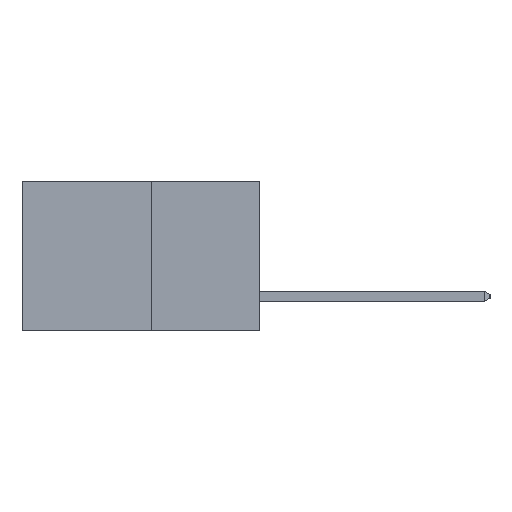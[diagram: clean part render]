
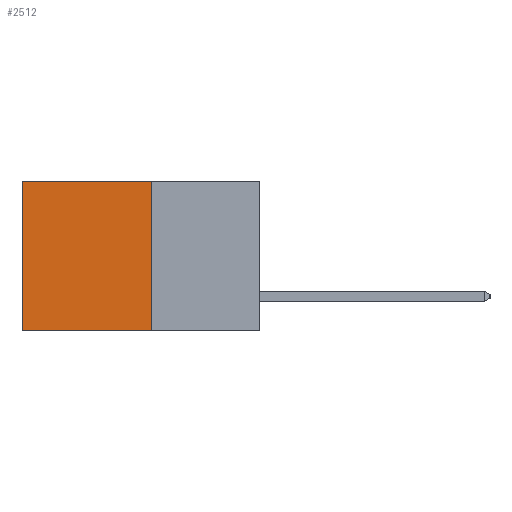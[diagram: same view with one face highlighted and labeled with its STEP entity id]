
A CAD part, left-side view. The second image highlights one B-rep face of the part: STEP entity #2512.
In plain terms, the highlighted planar face has unit normal (-1, 0, 0).
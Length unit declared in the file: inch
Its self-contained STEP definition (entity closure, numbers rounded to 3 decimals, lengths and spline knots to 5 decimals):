
#58 = VERTEX_POINT ( 'NONE', #10899 ) ;
#390 = ORIENTED_EDGE ( 'NONE', *, *, #5975, .T. ) ;
#1043 = VERTEX_POINT ( 'NONE', #5877 ) ;
#1537 = EDGE_CURVE ( 'NONE', #4087, #1043, #2656, .T. ) ;
#1836 = CARTESIAN_POINT ( 'NONE',  ( 0.277, 0.27, -0.37 ) ) ;
#1983 = FACE_OUTER_BOUND ( 'NONE', #2102, .T. ) ;
#2102 = EDGE_LOOP ( 'NONE', ( #390, #5267, #7483, #3284 ) ) ;
#2512 = ADVANCED_FACE ( 'NONE', ( #1983 ), #8039, .F. ) ;
#2656 = LINE ( 'NONE', #6248, #6930 ) ;
#3281 = VECTOR ( 'NONE', #5648, 39.37008 ) ;
#3284 = ORIENTED_EDGE ( 'NONE', *, *, #8163, .T. ) ;
#3298 = CARTESIAN_POINT ( 'NONE',  ( 0.277, 0.27, 0. ) ) ;
#3311 = DIRECTION ( 'NONE',  ( 0., 0., -1. ) ) ;
#3386 = VECTOR ( 'NONE', #7865, 39.37008 ) ;
#3498 = CARTESIAN_POINT ( 'NONE',  ( 0.277, 0.27, -0.37 ) ) ;
#4087 = VERTEX_POINT ( 'NONE', #1836 ) ;
#4350 = AXIS2_PLACEMENT_3D ( 'NONE', #7510, #7957, #7754 ) ;
#5099 = LINE ( 'NONE', #3498, #9199 ) ;
#5267 = ORIENTED_EDGE ( 'NONE', *, *, #1537, .F. ) ;
#5377 = LINE ( 'NONE', #7908, #3386 ) ;
#5546 = LINE ( 'NONE', #5722, #3281 ) ;
#5648 = DIRECTION ( 'NONE',  ( 0., 0., -1. ) ) ;
#5722 = CARTESIAN_POINT ( 'NONE',  ( 0.277, 0.59, -0.37 ) ) ;
#5877 = CARTESIAN_POINT ( 'NONE',  ( 0.277, 0.59, -0.37 ) ) ;
#5975 = EDGE_CURVE ( 'NONE', #58, #1043, #5546, .T. ) ;
#6049 = DIRECTION ( 'NONE',  ( 0., 1., 0. ) ) ;
#6248 = CARTESIAN_POINT ( 'NONE',  ( 0.277, 0.27, -0.37 ) ) ;
#6930 = VECTOR ( 'NONE', #6049, 39.37008 ) ;
#7289 = EDGE_CURVE ( 'NONE', #9110, #4087, #5099, .T. ) ;
#7483 = ORIENTED_EDGE ( 'NONE', *, *, #7289, .F. ) ;
#7510 = CARTESIAN_POINT ( 'NONE',  ( 0.277, 0.27, -0.37 ) ) ;
#7754 = DIRECTION ( 'NONE',  ( 0., 0., -1. ) ) ;
#7865 = DIRECTION ( 'NONE',  ( 0., 1., 0. ) ) ;
#7908 = CARTESIAN_POINT ( 'NONE',  ( 0.277, 0.27, 0. ) ) ;
#7957 = DIRECTION ( 'NONE',  ( 1., 0., 0. ) ) ;
#8039 = PLANE ( 'NONE',  #4350 ) ;
#8163 = EDGE_CURVE ( 'NONE', #9110, #58, #5377, .T. ) ;
#9110 = VERTEX_POINT ( 'NONE', #3298 ) ;
#9199 = VECTOR ( 'NONE', #3311, 39.37008 ) ;
#10899 = CARTESIAN_POINT ( 'NONE',  ( 0.277, 0.59, 0. ) ) ;
